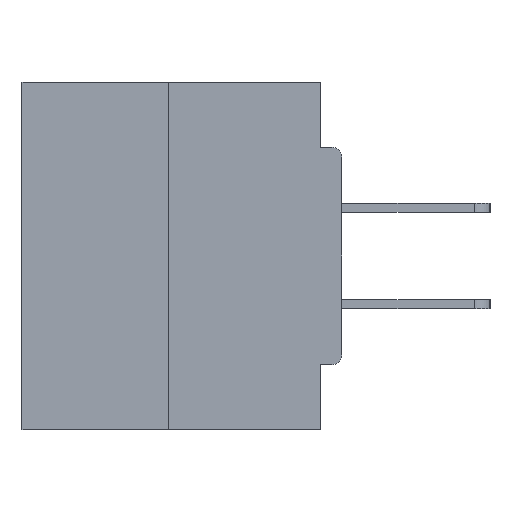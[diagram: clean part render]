
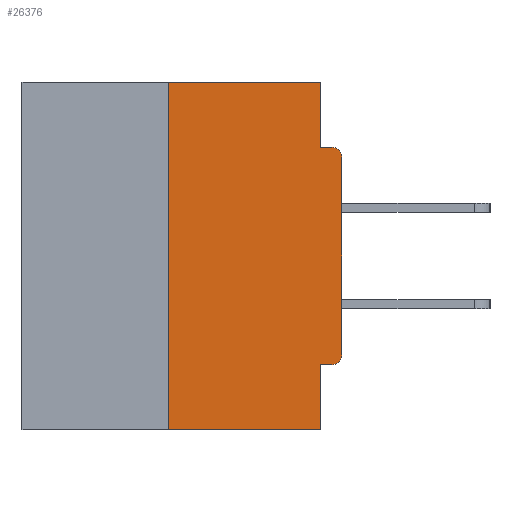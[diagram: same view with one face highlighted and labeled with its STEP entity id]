
A CAD part, left-side view. The second image highlights one B-rep face of the part: STEP entity #26376.
In plain terms, the highlighted planar face has unit normal (-1, 0, 0).
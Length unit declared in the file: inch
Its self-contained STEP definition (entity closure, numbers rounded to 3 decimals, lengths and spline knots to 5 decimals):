
#400 = VECTOR ( 'NONE', #24720, 39.37008 ) ;
#421 = CARTESIAN_POINT ( 'NONE',  ( 0., 0.031, -0.5 ) ) ;
#1999 = LINE ( 'NONE', #15345, #2530 ) ;
#2327 = VECTOR ( 'NONE', #6317, 39.37008 ) ;
#2389 = AXIS2_PLACEMENT_3D ( 'NONE', #28395, #34496, #29179 ) ;
#2466 = CARTESIAN_POINT ( 'NONE',  ( 0., 0.46, 0. ) ) ;
#2530 = VECTOR ( 'NONE', #13357, 39.37008 ) ;
#2755 = DIRECTION ( 'NONE',  ( 0., -1., 0. ) ) ;
#2978 = ORIENTED_EDGE ( 'NONE', *, *, #29992, .T. ) ;
#3063 = CARTESIAN_POINT ( 'NONE',  ( 0., 0.015, -0.4065 ) ) ;
#3085 = ORIENTED_EDGE ( 'NONE', *, *, #28307, .T. ) ;
#3262 = VECTOR ( 'NONE', #17046, 39.37008 ) ;
#4288 = CARTESIAN_POINT ( 'NONE',  ( 0., 0.25, -0.5 ) ) ;
#4314 = VECTOR ( 'NONE', #17427, 39.37008 ) ;
#5068 = ORIENTED_EDGE ( 'NONE', *, *, #20823, .F. ) ;
#5794 = EDGE_CURVE ( 'NONE', #29549, #17671, #22880, .T. ) ;
#6317 = DIRECTION ( 'NONE',  ( 0., -1., 0. ) ) ;
#6854 = EDGE_CURVE ( 'NONE', #29549, #25548, #12138, .T. ) ;
#7221 = DIRECTION ( 'NONE',  ( 0., 0., -1. ) ) ;
#9181 = LINE ( 'NONE', #12534, #400 ) ;
#9624 = CARTESIAN_POINT ( 'NONE',  ( 0., 0.015, -0.0935 ) ) ;
#11056 = FACE_OUTER_BOUND ( 'NONE', #26404, .T. ) ;
#11854 = CIRCLE ( 'NONE', #34197, 0.015 ) ;
#12138 = LINE ( 'NONE', #35885, #4314 ) ;
#12534 = CARTESIAN_POINT ( 'NONE',  ( 0., 0., 0. ) ) ;
#13346 = DIRECTION ( 'NONE',  ( 1., 0., 0. ) ) ;
#13357 = DIRECTION ( 'NONE',  ( 0., -1., 0. ) ) ;
#13535 = VECTOR ( 'NONE', #15930, 39.37008 ) ;
#14273 = CARTESIAN_POINT ( 'NONE',  ( 0., 0.031, -0.0935 ) ) ;
#14281 = CARTESIAN_POINT ( 'NONE',  ( 0., 0.015, -0.1085 ) ) ;
#14514 = LINE ( 'NONE', #27809, #2327 ) ;
#15070 = EDGE_CURVE ( 'NONE', #34390, #18761, #14514, .T. ) ;
#15131 = ORIENTED_EDGE ( 'NONE', *, *, #26679, .F. ) ;
#15250 = ORIENTED_EDGE ( 'NONE', *, *, #31047, .F. ) ;
#15345 = CARTESIAN_POINT ( 'NONE',  ( 0., 0., -0.0935 ) ) ;
#15930 = DIRECTION ( 'NONE',  ( 0., 0., 1. ) ) ;
#16289 = CARTESIAN_POINT ( 'NONE',  ( 0., 0.031, -0.4065 ) ) ;
#17046 = DIRECTION ( 'NONE',  ( 0., 0., -1. ) ) ;
#17314 = EDGE_CURVE ( 'NONE', #31697, #21142, #11854, .T. ) ;
#17386 = DIRECTION ( 'NONE',  ( 0., 0., -1. ) ) ;
#17427 = DIRECTION ( 'NONE',  ( 0., 1., 0. ) ) ;
#17671 = VERTEX_POINT ( 'NONE', #22921 ) ;
#18761 = VERTEX_POINT ( 'NONE', #39604 ) ;
#19122 = CARTESIAN_POINT ( 'NONE',  ( 0., 0.25, 0. ) ) ;
#19706 = ORIENTED_EDGE ( 'NONE', *, *, #6854, .F. ) ;
#19762 = LINE ( 'NONE', #421, #37132 ) ;
#20148 = CARTESIAN_POINT ( 'NONE',  ( 0., 0.031, 0. ) ) ;
#20823 = EDGE_CURVE ( 'NONE', #18761, #32354, #39468, .T. ) ;
#21142 = VERTEX_POINT ( 'NONE', #9624 ) ;
#21201 = CARTESIAN_POINT ( 'NONE',  ( 0., 0.46, -0.5 ) ) ;
#22880 = CIRCLE ( 'NONE', #2389, 0.015 ) ;
#22921 = CARTESIAN_POINT ( 'NONE',  ( 0., 0., -0.3915 ) ) ;
#22926 = ORIENTED_EDGE ( 'NONE', *, *, #15070, .F. ) ;
#24077 = ORIENTED_EDGE ( 'NONE', *, *, #17314, .T. ) ;
#24245 = CARTESIAN_POINT ( 'NONE',  ( 0., 0.25, 0. ) ) ;
#24720 = DIRECTION ( 'NONE',  ( 0., 0., 1. ) ) ;
#25548 = VERTEX_POINT ( 'NONE', #16289 ) ;
#26376 = ADVANCED_FACE ( 'NONE', ( #11056 ), #36939, .F. ) ;
#26404 = EDGE_LOOP ( 'NONE', ( #22926, #27455, #2978, #15131, #19706, #32799, #3085, #24077, #15250, #5068 ) ) ;
#26624 = EDGE_CURVE ( 'NONE', #35622, #34390, #36185, .T. ) ;
#26679 = EDGE_CURVE ( 'NONE', #25548, #28874, #19762, .T. ) ;
#27455 = ORIENTED_EDGE ( 'NONE', *, *, #26624, .F. ) ;
#27809 = CARTESIAN_POINT ( 'NONE',  ( 0., 0.46, 0. ) ) ;
#28307 = EDGE_CURVE ( 'NONE', #17671, #31697, #9181, .T. ) ;
#28395 = CARTESIAN_POINT ( 'NONE',  ( 0., 0.015, -0.3915 ) ) ;
#28874 = VERTEX_POINT ( 'NONE', #32334 ) ;
#29179 = DIRECTION ( 'NONE',  ( 0., 0., -1. ) ) ;
#29549 = VERTEX_POINT ( 'NONE', #3063 ) ;
#29992 = EDGE_CURVE ( 'NONE', #35622, #28874, #38381, .T. ) ;
#31047 = EDGE_CURVE ( 'NONE', #32354, #21142, #1999, .T. ) ;
#31697 = VERTEX_POINT ( 'NONE', #32537 ) ;
#32334 = CARTESIAN_POINT ( 'NONE',  ( 0., 0.031, -0.5 ) ) ;
#32354 = VERTEX_POINT ( 'NONE', #14273 ) ;
#32537 = CARTESIAN_POINT ( 'NONE',  ( 0., 0., -0.1085 ) ) ;
#32799 = ORIENTED_EDGE ( 'NONE', *, *, #5794, .T. ) ;
#33888 = AXIS2_PLACEMENT_3D ( 'NONE', #2466, #13346, #7221 ) ;
#34197 = AXIS2_PLACEMENT_3D ( 'NONE', #14281, #35854, #17386 ) ;
#34390 = VERTEX_POINT ( 'NONE', #24245 ) ;
#34496 = DIRECTION ( 'NONE',  ( -1., 0., 0. ) ) ;
#34497 = DIRECTION ( 'NONE',  ( 0., 0., -1. ) ) ;
#35622 = VERTEX_POINT ( 'NONE', #4288 ) ;
#35854 = DIRECTION ( 'NONE',  ( -1., 0., 0. ) ) ;
#35885 = CARTESIAN_POINT ( 'NONE',  ( 0., 0., -0.4065 ) ) ;
#36185 = LINE ( 'NONE', #19122, #13535 ) ;
#36939 = PLANE ( 'NONE',  #33888 ) ;
#37132 = VECTOR ( 'NONE', #34497, 39.37008 ) ;
#38381 = LINE ( 'NONE', #21201, #39351 ) ;
#39351 = VECTOR ( 'NONE', #2755, 39.37008 ) ;
#39468 = LINE ( 'NONE', #20148, #3262 ) ;
#39604 = CARTESIAN_POINT ( 'NONE',  ( 0., 0.031, 0. ) ) ;
